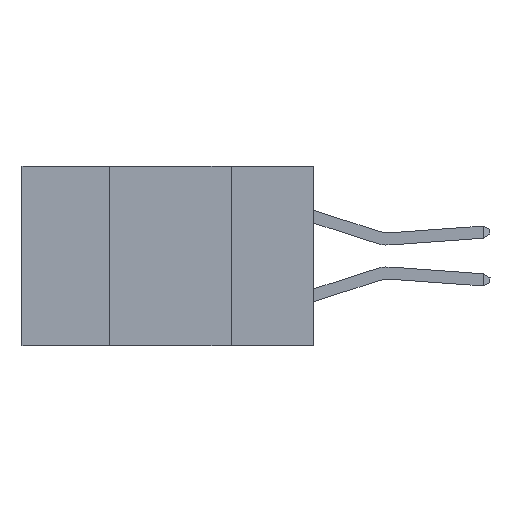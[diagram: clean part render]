
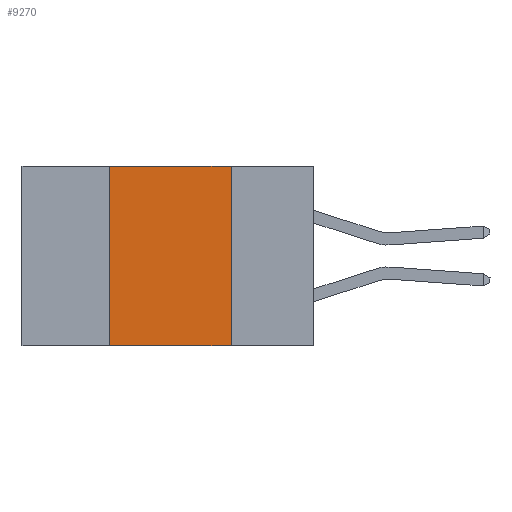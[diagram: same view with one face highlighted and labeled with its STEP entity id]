
A CAD part, left-side view. The second image highlights one B-rep face of the part: STEP entity #9270.
In plain terms, the highlighted planar face has unit normal (-1, 0, 0).
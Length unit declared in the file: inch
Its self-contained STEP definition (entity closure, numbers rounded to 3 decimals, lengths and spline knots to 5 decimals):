
#389 = CARTESIAN_POINT ( 'NONE',  ( 0., 0.6, 0. ) ) ;
#570 = VERTEX_POINT ( 'NONE', #1648 ) ;
#1648 = CARTESIAN_POINT ( 'NONE',  ( 0., 0.17, -0.37 ) ) ;
#1955 = DIRECTION ( 'NONE',  ( 0., -1., 0. ) ) ;
#2087 = ORIENTED_EDGE ( 'NONE', *, *, #4554, .F. ) ;
#2236 = AXIS2_PLACEMENT_3D ( 'NONE', #389, #6455, #5669 ) ;
#2279 = LINE ( 'NONE', #8968, #6185 ) ;
#2525 = LINE ( 'NONE', #4928, #4053 ) ;
#2556 = PLANE ( 'NONE',  #2236 ) ;
#3305 = VERTEX_POINT ( 'NONE', #9673 ) ;
#3451 = EDGE_CURVE ( 'NONE', #8446, #570, #5631, .T. ) ;
#3863 = EDGE_CURVE ( 'NONE', #4577, #3305, #7978, .T. ) ;
#4053 = VECTOR ( 'NONE', #7359, 39.37008 ) ;
#4554 = EDGE_CURVE ( 'NONE', #8446, #4577, #2279, .T. ) ;
#4577 = VERTEX_POINT ( 'NONE', #5454 ) ;
#4928 = CARTESIAN_POINT ( 'NONE',  ( 0., 0.17, 0. ) ) ;
#5222 = FACE_OUTER_BOUND ( 'NONE', #8180, .T. ) ;
#5249 = DIRECTION ( 'NONE',  ( 0., 0., 1. ) ) ;
#5454 = CARTESIAN_POINT ( 'NONE',  ( 0., 0.42, 0. ) ) ;
#5555 = ORIENTED_EDGE ( 'NONE', *, *, #6769, .F. ) ;
#5631 = LINE ( 'NONE', #5637, #7752 ) ;
#5637 = CARTESIAN_POINT ( 'NONE',  ( 0., 0.6, -0.37 ) ) ;
#5669 = DIRECTION ( 'NONE',  ( 0., 0., -1. ) ) ;
#5856 = ORIENTED_EDGE ( 'NONE', *, *, #3451, .T. ) ;
#6019 = CARTESIAN_POINT ( 'NONE',  ( 0., 0.6, 0. ) ) ;
#6185 = VECTOR ( 'NONE', #5249, 39.37008 ) ;
#6455 = DIRECTION ( 'NONE',  ( 1., 0., 0. ) ) ;
#6769 = EDGE_CURVE ( 'NONE', #3305, #570, #2525, .T. ) ;
#7359 = DIRECTION ( 'NONE',  ( 0., 0., -1. ) ) ;
#7752 = VECTOR ( 'NONE', #1955, 39.37008 ) ;
#7873 = VECTOR ( 'NONE', #8301, 39.37008 ) ;
#7978 = LINE ( 'NONE', #6019, #7873 ) ;
#7985 = CARTESIAN_POINT ( 'NONE',  ( 0., 0.42, -0.37 ) ) ;
#8180 = EDGE_LOOP ( 'NONE', ( #5555, #8198, #2087, #5856 ) ) ;
#8198 = ORIENTED_EDGE ( 'NONE', *, *, #3863, .F. ) ;
#8301 = DIRECTION ( 'NONE',  ( 0., -1., 0. ) ) ;
#8446 = VERTEX_POINT ( 'NONE', #7985 ) ;
#8968 = CARTESIAN_POINT ( 'NONE',  ( 0., 0.42, 0. ) ) ;
#9270 = ADVANCED_FACE ( 'NONE', ( #5222 ), #2556, .F. ) ;
#9673 = CARTESIAN_POINT ( 'NONE',  ( 0., 0.17, 0. ) ) ;
